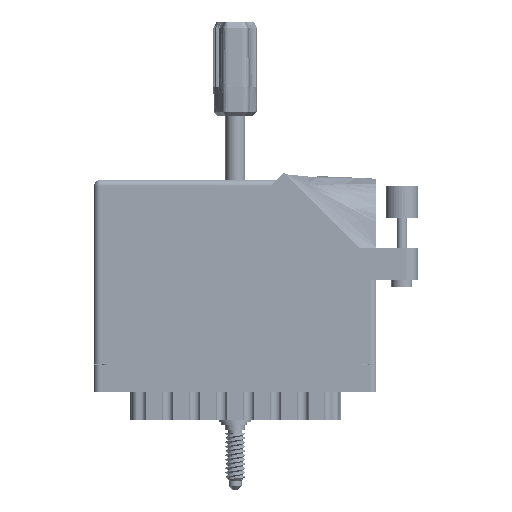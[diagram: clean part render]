
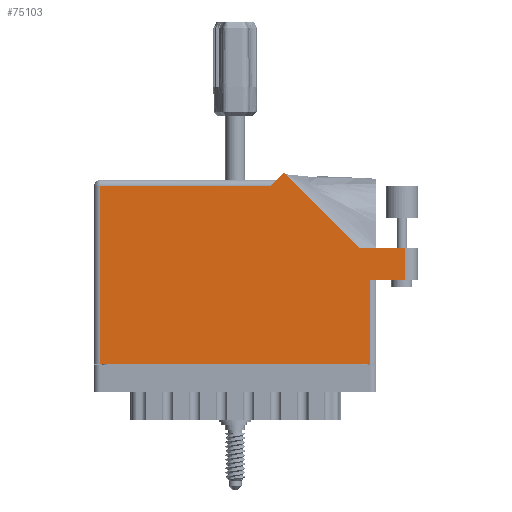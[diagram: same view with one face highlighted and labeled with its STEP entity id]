
A CAD part, front view. The second image highlights one B-rep face of the part: STEP entity #75103.
In plain terms, the highlighted face is planar.
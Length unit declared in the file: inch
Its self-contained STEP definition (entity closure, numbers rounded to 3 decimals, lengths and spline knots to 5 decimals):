
#1914 = CARTESIAN_POINT ( 'NONE',  ( 0., 0., 0. ) ) ;
#2588 = EDGE_CURVE ( 'NONE', #86770, #12808, #53838, .T. ) ;
#4510 = ORIENTED_EDGE ( 'NONE', *, *, #2588, .T. ) ;
#7297 = LINE ( 'NONE', #77231, #19217 ) ;
#8028 = VERTEX_POINT ( 'NONE', #48299 ) ;
#8311 = VERTEX_POINT ( 'NONE', #9186 ) ;
#9186 = CARTESIAN_POINT ( 'NONE',  ( 0.062, 0., 0. ) ) ;
#10785 = CARTESIAN_POINT ( 'NONE',  ( 1.758, 1.775, 0. ) ) ;
#11857 = CARTESIAN_POINT ( 'NONE',  ( 1.82871, 1.84571, 0. ) ) ;
#12011 = DIRECTION ( 'NONE',  ( -1., 0., 0. ) ) ;
#12158 = PLANE ( 'NONE',  #22383 ) ;
#12808 = VERTEX_POINT ( 'NONE', #47893 ) ;
#12883 = VERTEX_POINT ( 'NONE', #63220 ) ;
#16662 = CARTESIAN_POINT ( 'NONE',  ( 2.993, 1.122, 0. ) ) ;
#16981 = EDGE_CURVE ( 'NONE', #8028, #12883, #29909, .T. ) ;
#18520 = ORIENTED_EDGE ( 'NONE', *, *, #54310, .T. ) ;
#18827 = ORIENTED_EDGE ( 'NONE', *, *, #57010, .T. ) ;
#19217 = VECTOR ( 'NONE', #69082, 39.37008 ) ;
#21126 = CARTESIAN_POINT ( 'NONE',  ( 2.718, 0.815, 0. ) ) ;
#21862 = VECTOR ( 'NONE', #23745, 39.37008 ) ;
#22383 = AXIS2_PLACEMENT_3D ( 'NONE', #81359, #39489, #33658 ) ;
#23745 = DIRECTION ( 'NONE',  ( -1., 0., 0. ) ) ;
#24560 = VECTOR ( 'NONE', #71067, 39.37008 ) ;
#24740 = DIRECTION ( 'NONE',  ( -0.707, -0.707, 0. ) ) ;
#29909 = LINE ( 'NONE', #63801, #24560 ) ;
#30055 = CARTESIAN_POINT ( 'NONE',  ( 0.062, 1.713, 0. ) ) ;
#31938 = VERTEX_POINT ( 'NONE', #40472 ) ;
#32003 = CARTESIAN_POINT ( 'NONE',  ( 0., 1.713, 0. ) ) ;
#32852 = VECTOR ( 'NONE', #50313, 39.37008 ) ;
#33658 = DIRECTION ( 'NONE',  ( -1., 0., 0. ) ) ;
#34514 = ORIENTED_EDGE ( 'NONE', *, *, #34527, .T. ) ;
#34527 = EDGE_CURVE ( 'NONE', #31938, #68543, #34913, .T. ) ;
#34913 = LINE ( 'NONE', #43795, #21862 ) ;
#37784 = ORIENTED_EDGE ( 'NONE', *, *, #16981, .T. ) ;
#37919 = ORIENTED_EDGE ( 'NONE', *, *, #38331, .T. ) ;
#38189 = LINE ( 'NONE', #21126, #73791 ) ;
#38331 = EDGE_CURVE ( 'NONE', #68543, #86770, #7297, .T. ) ;
#39324 = EDGE_CURVE ( 'NONE', #60821, #31938, #60166, .T. ) ;
#39489 = DIRECTION ( 'NONE',  ( 0., 0., -1. ) ) ;
#40472 = CARTESIAN_POINT ( 'NONE',  ( 2.993, 1.122, 0. ) ) ;
#42909 = VECTOR ( 'NONE', #12011, 39.37008 ) ;
#43795 = CARTESIAN_POINT ( 'NONE',  ( 3.118, 1.122, 0. ) ) ;
#47893 = CARTESIAN_POINT ( 'NONE',  ( 1.696, 1.713, 0. ) ) ;
#48299 = CARTESIAN_POINT ( 'NONE',  ( 2.656, 0., 0. ) ) ;
#48528 = VECTOR ( 'NONE', #64899, 39.37008 ) ;
#50313 = DIRECTION ( 'NONE',  ( 1., 0., 0. ) ) ;
#51360 = CARTESIAN_POINT ( 'NONE',  ( 0.062, 0., 0. ) ) ;
#53838 = LINE ( 'NONE', #10785, #87192 ) ;
#54310 = EDGE_CURVE ( 'NONE', #12883, #60821, #38189, .T. ) ;
#55021 = LINE ( 'NONE', #51360, #48528 ) ;
#57010 = EDGE_CURVE ( 'NONE', #65803, #8311, #55021, .T. ) ;
#59828 = CARTESIAN_POINT ( 'NONE',  ( 2.993, 0.815, 0. ) ) ;
#60166 = LINE ( 'NONE', #16662, #69851 ) ;
#60404 = EDGE_LOOP ( 'NONE', ( #18520, #82427, #34514, #37919, #4510, #63098, #18827, #66821, #37784 ) ) ;
#60821 = VERTEX_POINT ( 'NONE', #59828 ) ;
#63098 = ORIENTED_EDGE ( 'NONE', *, *, #89480, .T. ) ;
#63220 = CARTESIAN_POINT ( 'NONE',  ( 2.656, 0.815, 0. ) ) ;
#63800 = FACE_OUTER_BOUND ( 'NONE', #60404, .T. ) ;
#63801 = CARTESIAN_POINT ( 'NONE',  ( 2.656, 0.815, 0. ) ) ;
#64899 = DIRECTION ( 'NONE',  ( 0., -1., 0. ) ) ;
#65803 = VERTEX_POINT ( 'NONE', #30055 ) ;
#66821 = ORIENTED_EDGE ( 'NONE', *, *, #83280, .T. ) ;
#67443 = LINE ( 'NONE', #1914, #32852 ) ;
#68543 = VERTEX_POINT ( 'NONE', #69692 ) ;
#69082 = DIRECTION ( 'NONE',  ( -0.707, 0.707, 0. ) ) ;
#69475 = DIRECTION ( 'NONE',  ( 1., 0., 0. ) ) ;
#69692 = CARTESIAN_POINT ( 'NONE',  ( 2.55242, 1.122, 0. ) ) ;
#69851 = VECTOR ( 'NONE', #72314, 39.37008 ) ;
#71067 = DIRECTION ( 'NONE',  ( 0., 1., 0. ) ) ;
#72314 = DIRECTION ( 'NONE',  ( 0., 1., 0. ) ) ;
#73791 = VECTOR ( 'NONE', #69475, 39.37008 ) ;
#75103 = ADVANCED_FACE ( 'NONE', ( #63800 ), #12158, .F. ) ;
#77231 = CARTESIAN_POINT ( 'NONE',  ( 2.55242, 1.122, 0. ) ) ;
#81359 = CARTESIAN_POINT ( 'NONE',  ( 0., 1.775, 0. ) ) ;
#81716 = LINE ( 'NONE', #32003, #42909 ) ;
#82427 = ORIENTED_EDGE ( 'NONE', *, *, #39324, .T. ) ;
#83280 = EDGE_CURVE ( 'NONE', #8311, #8028, #67443, .T. ) ;
#86770 = VERTEX_POINT ( 'NONE', #11857 ) ;
#87192 = VECTOR ( 'NONE', #24740, 39.37008 ) ;
#89480 = EDGE_CURVE ( 'NONE', #12808, #65803, #81716, .T. ) ;
